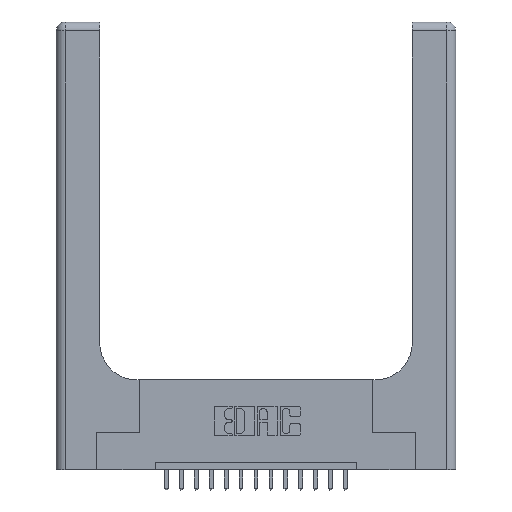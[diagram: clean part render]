
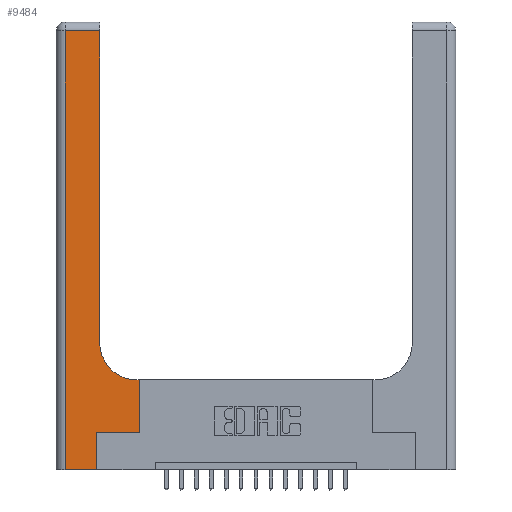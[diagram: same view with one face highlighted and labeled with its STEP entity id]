
A CAD part, top view. The second image highlights one B-rep face of the part: STEP entity #9484.
In plain terms, the highlighted planar face has unit normal (0, 0, 1).
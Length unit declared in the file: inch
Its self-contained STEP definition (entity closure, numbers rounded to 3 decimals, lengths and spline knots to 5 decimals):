
#546 = DIRECTION ( 'NONE',  ( -1., 0., 0. ) ) ;
#673 = LINE ( 'NONE', #11211, #16414 ) ;
#1049 = ORIENTED_EDGE ( 'NONE', *, *, #8208, .T. ) ;
#1480 = DIRECTION ( 'NONE',  ( 0., 1., 0. ) ) ;
#1642 = VERTEX_POINT ( 'NONE', #13066 ) ;
#1986 = EDGE_CURVE ( 'NONE', #10407, #17966, #673, .T. ) ;
#2167 = ORIENTED_EDGE ( 'NONE', *, *, #17970, .T. ) ;
#2607 = CARTESIAN_POINT ( 'NONE',  ( 0.5415, 0.6, 0.37 ) ) ;
#3030 = ORIENTED_EDGE ( 'NONE', *, *, #12063, .T. ) ;
#3089 = VECTOR ( 'NONE', #17993, 39.37008 ) ;
#3149 = CIRCLE ( 'NONE', #15063, 0.25 ) ;
#3162 = VECTOR ( 'NONE', #546, 39.37008 ) ;
#3654 = VECTOR ( 'NONE', #5457, 39.37008 ) ;
#3902 = VERTEX_POINT ( 'NONE', #6111 ) ;
#4555 = ORIENTED_EDGE ( 'NONE', *, *, #14565, .T. ) ;
#4874 = DIRECTION ( 'NONE',  ( 0., 0., -1. ) ) ;
#5053 = DIRECTION ( 'NONE',  ( 1., 0., 0. ) ) ;
#5112 = DIRECTION ( 'NONE',  ( -1., 0., 0. ) ) ;
#5400 = CARTESIAN_POINT ( 'NONE',  ( 0., 2.94, 0.37 ) ) ;
#5457 = DIRECTION ( 'NONE',  ( -1., 0., 0. ) ) ;
#5924 = EDGE_CURVE ( 'NONE', #10132, #18540, #10944, .T. ) ;
#5958 = FACE_OUTER_BOUND ( 'NONE', #17184, .T. ) ;
#6111 = CARTESIAN_POINT ( 'NONE',  ( 0.2915, 2.94, 0.37 ) ) ;
#6421 = CARTESIAN_POINT ( 'NONE',  ( 0.269, 0.25, 0.37 ) ) ;
#6542 = PLANE ( 'NONE',  #15599 ) ;
#6665 = CARTESIAN_POINT ( 'NONE',  ( 0., 3., 0.37 ) ) ;
#7455 = CARTESIAN_POINT ( 'NONE',  ( 0.269, 0., 0.37 ) ) ;
#7633 = CARTESIAN_POINT ( 'NONE',  ( 0.269, 0.25, 0.37 ) ) ;
#7685 = VECTOR ( 'NONE', #1480, 39.37008 ) ;
#8208 = EDGE_CURVE ( 'NONE', #14440, #10407, #15354, .T. ) ;
#8404 = CARTESIAN_POINT ( 'NONE',  ( 0.5585, 0.25, 0.37 ) ) ;
#8712 = LINE ( 'NONE', #7633, #17800 ) ;
#8788 = CARTESIAN_POINT ( 'NONE',  ( 0.06, 3., 0.37 ) ) ;
#9039 = ORIENTED_EDGE ( 'NONE', *, *, #17514, .T. ) ;
#9484 = ADVANCED_FACE ( 'NONE', ( #5958 ), #6542, .F. ) ;
#9640 = DIRECTION ( 'NONE',  ( 0., 1., 0. ) ) ;
#10132 = VERTEX_POINT ( 'NONE', #8404 ) ;
#10407 = VERTEX_POINT ( 'NONE', #7455 ) ;
#10548 = LINE ( 'NONE', #5400, #3654 ) ;
#10592 = VECTOR ( 'NONE', #12118, 39.37008 ) ;
#10718 = CARTESIAN_POINT ( 'NONE',  ( 0.5585, 0.6, 0.37 ) ) ;
#10944 = LINE ( 'NONE', #16565, #3089 ) ;
#11211 = CARTESIAN_POINT ( 'NONE',  ( 0.269, 0., 0.37 ) ) ;
#11575 = ORIENTED_EDGE ( 'NONE', *, *, #11796, .T. ) ;
#11755 = ORIENTED_EDGE ( 'NONE', *, *, #14509, .T. ) ;
#11796 = EDGE_CURVE ( 'NONE', #3902, #12201, #10548, .T. ) ;
#11841 = VECTOR ( 'NONE', #17668, 39.37008 ) ;
#12063 = EDGE_CURVE ( 'NONE', #18540, #13755, #17339, .T. ) ;
#12118 = DIRECTION ( 'NONE',  ( 1., 0., 0. ) ) ;
#12201 = VERTEX_POINT ( 'NONE', #14552 ) ;
#12431 = ORIENTED_EDGE ( 'NONE', *, *, #1986, .T. ) ;
#13066 = CARTESIAN_POINT ( 'NONE',  ( 0.2915, 0.85, 0.37 ) ) ;
#13649 = LINE ( 'NONE', #16108, #7685 ) ;
#13755 = VERTEX_POINT ( 'NONE', #2607 ) ;
#13781 = ORIENTED_EDGE ( 'NONE', *, *, #5924, .T. ) ;
#14335 = LINE ( 'NONE', #8788, #11841 ) ;
#14440 = VERTEX_POINT ( 'NONE', #14535 ) ;
#14509 = EDGE_CURVE ( 'NONE', #1642, #3902, #13649, .T. ) ;
#14535 = CARTESIAN_POINT ( 'NONE',  ( 0.06, 0., 0.37 ) ) ;
#14552 = CARTESIAN_POINT ( 'NONE',  ( 0.06, 2.94, 0.37 ) ) ;
#14565 = EDGE_CURVE ( 'NONE', #12201, #14440, #14335, .T. ) ;
#15063 = AXIS2_PLACEMENT_3D ( 'NONE', #18110, #4874, #5053 ) ;
#15102 = CARTESIAN_POINT ( 'NONE',  ( 0.2915, 0.6, 0.37 ) ) ;
#15354 = LINE ( 'NONE', #16468, #10592 ) ;
#15599 = AXIS2_PLACEMENT_3D ( 'NONE', #6665, #16747, #5112 ) ;
#16108 = CARTESIAN_POINT ( 'NONE',  ( 0.2915, 3., 0.37 ) ) ;
#16414 = VECTOR ( 'NONE', #9640, 39.37008 ) ;
#16468 = CARTESIAN_POINT ( 'NONE',  ( 0., 0., 0.37 ) ) ;
#16565 = CARTESIAN_POINT ( 'NONE',  ( 0.5585, 0.25, 0.37 ) ) ;
#16747 = DIRECTION ( 'NONE',  ( 0., 0., -1. ) ) ;
#17184 = EDGE_LOOP ( 'NONE', ( #11755, #11575, #4555, #1049, #12431, #9039, #13781, #3030, #2167 ) ) ;
#17339 = LINE ( 'NONE', #15102, #3162 ) ;
#17514 = EDGE_CURVE ( 'NONE', #17966, #10132, #8712, .T. ) ;
#17668 = DIRECTION ( 'NONE',  ( 0., -1., 0. ) ) ;
#17800 = VECTOR ( 'NONE', #18393, 39.37008 ) ;
#17966 = VERTEX_POINT ( 'NONE', #6421 ) ;
#17970 = EDGE_CURVE ( 'NONE', #13755, #1642, #3149, .T. ) ;
#17993 = DIRECTION ( 'NONE',  ( 0., 1., 0. ) ) ;
#18110 = CARTESIAN_POINT ( 'NONE',  ( 0.5415, 0.85, 0.37 ) ) ;
#18393 = DIRECTION ( 'NONE',  ( 1., 0., 0. ) ) ;
#18540 = VERTEX_POINT ( 'NONE', #10718 ) ;
